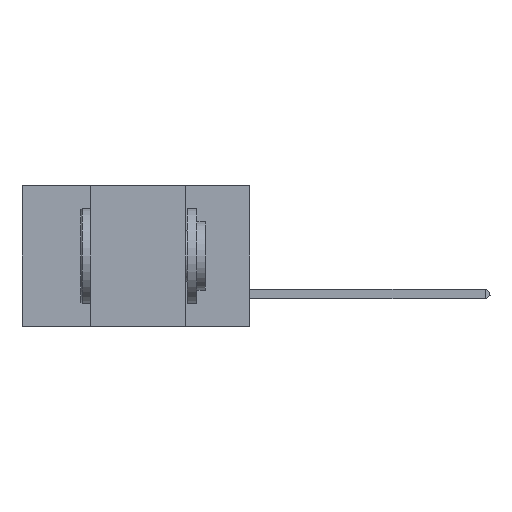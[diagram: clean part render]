
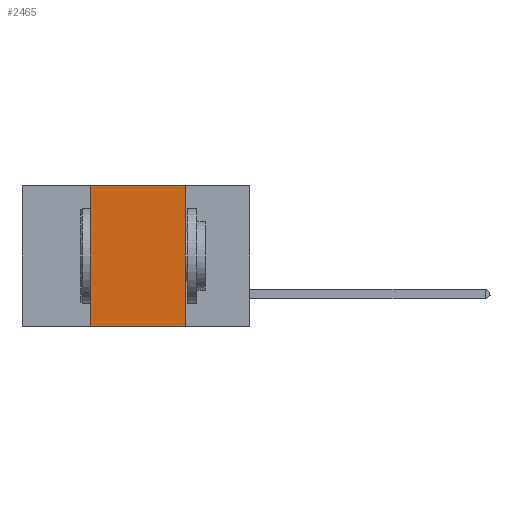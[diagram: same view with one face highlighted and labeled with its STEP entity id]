
A CAD part, left-side view. The second image highlights one B-rep face of the part: STEP entity #2465.
In plain terms, the highlighted planar face has unit normal (-1, 0, 0).
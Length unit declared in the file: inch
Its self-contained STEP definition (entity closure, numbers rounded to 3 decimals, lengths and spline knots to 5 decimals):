
#138 = DIRECTION ( 'NONE',  ( 0., 0., -1. ) ) ;
#362 = DIRECTION ( 'NONE',  ( 0., 0., 1. ) ) ;
#828 = CARTESIAN_POINT ( 'NONE',  ( 0., 0.6, 0. ) ) ;
#1365 = VERTEX_POINT ( 'NONE', #17752 ) ;
#2465 = ADVANCED_FACE ( 'NONE', ( #6943 ), #7967, .F. ) ;
#3121 = DIRECTION ( 'NONE',  ( 0., 0., -1. ) ) ;
#3702 = CARTESIAN_POINT ( 'NONE',  ( 0., 0.42, -0.37 ) ) ;
#3972 = VERTEX_POINT ( 'NONE', #17402 ) ;
#5390 = DIRECTION ( 'NONE',  ( 0., -1., 0. ) ) ;
#6031 = EDGE_LOOP ( 'NONE', ( #17844, #22899, #18188, #10276 ) ) ;
#6943 = FACE_OUTER_BOUND ( 'NONE', #6031, .T. ) ;
#6991 = EDGE_CURVE ( 'NONE', #11211, #1365, #13257, .T. ) ;
#7967 = PLANE ( 'NONE',  #11375 ) ;
#7973 = EDGE_CURVE ( 'NONE', #14124, #3972, #8515, .T. ) ;
#7992 = LINE ( 'NONE', #8126, #8275 ) ;
#8126 = CARTESIAN_POINT ( 'NONE',  ( 0., 0.42, 0. ) ) ;
#8275 = VECTOR ( 'NONE', #362, 39.37008 ) ;
#8508 = DIRECTION ( 'NONE',  ( 0., -1., 0. ) ) ;
#8515 = LINE ( 'NONE', #16745, #22072 ) ;
#10276 = ORIENTED_EDGE ( 'NONE', *, *, #7973, .T. ) ;
#10934 = EDGE_CURVE ( 'NONE', #14124, #11211, #7992, .T. ) ;
#11211 = VERTEX_POINT ( 'NONE', #14440 ) ;
#11375 = AXIS2_PLACEMENT_3D ( 'NONE', #11429, #18930, #138 ) ;
#11429 = CARTESIAN_POINT ( 'NONE',  ( 0., 0.6, 0. ) ) ;
#13257 = LINE ( 'NONE', #828, #16195 ) ;
#13955 = CARTESIAN_POINT ( 'NONE',  ( 0., 0.17, 0. ) ) ;
#14124 = VERTEX_POINT ( 'NONE', #3702 ) ;
#14440 = CARTESIAN_POINT ( 'NONE',  ( 0., 0.42, 0. ) ) ;
#16195 = VECTOR ( 'NONE', #8508, 39.37008 ) ;
#16358 = LINE ( 'NONE', #13955, #17225 ) ;
#16745 = CARTESIAN_POINT ( 'NONE',  ( 0., 0.6, -0.37 ) ) ;
#17225 = VECTOR ( 'NONE', #3121, 39.37008 ) ;
#17402 = CARTESIAN_POINT ( 'NONE',  ( 0., 0.17, -0.37 ) ) ;
#17752 = CARTESIAN_POINT ( 'NONE',  ( 0., 0.17, 0. ) ) ;
#17844 = ORIENTED_EDGE ( 'NONE', *, *, #19072, .F. ) ;
#18188 = ORIENTED_EDGE ( 'NONE', *, *, #10934, .F. ) ;
#18930 = DIRECTION ( 'NONE',  ( 1., 0., 0. ) ) ;
#19072 = EDGE_CURVE ( 'NONE', #1365, #3972, #16358, .T. ) ;
#22072 = VECTOR ( 'NONE', #5390, 39.37008 ) ;
#22899 = ORIENTED_EDGE ( 'NONE', *, *, #6991, .F. ) ;
